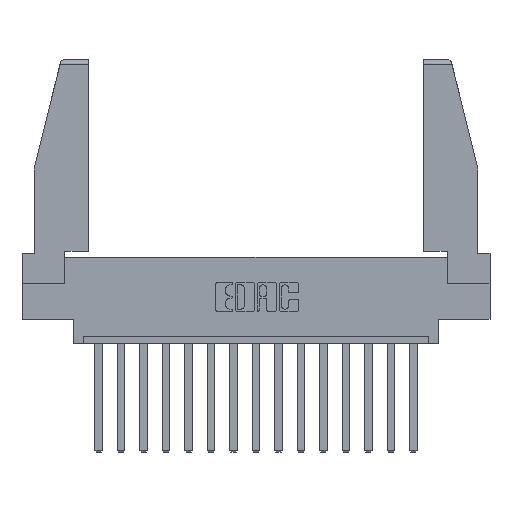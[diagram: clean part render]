
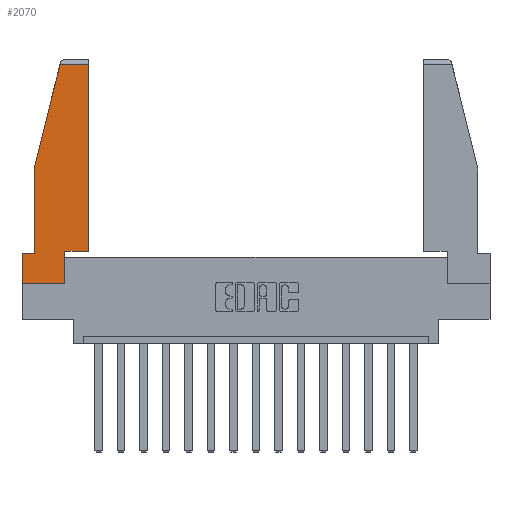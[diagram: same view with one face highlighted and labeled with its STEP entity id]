
A CAD part, top view. The second image highlights one B-rep face of the part: STEP entity #2070.
In plain terms, the highlighted planar face has unit normal (0, 0, 1).
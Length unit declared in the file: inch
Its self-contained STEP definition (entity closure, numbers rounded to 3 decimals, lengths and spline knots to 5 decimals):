
#109 = AXIS2_PLACEMENT_3D ( 'NONE', #7690, #15931, #11987 ) ;
#240 = EDGE_CURVE ( 'NONE', #331, #1604, #15141, .T. ) ;
#331 = VERTEX_POINT ( 'NONE', #11324 ) ;
#376 = LINE ( 'NONE', #4694, #9643 ) ;
#450 = DIRECTION ( 'NONE',  ( 1., 0., 0. ) ) ;
#595 = VERTEX_POINT ( 'NONE', #5426 ) ;
#1354 = VERTEX_POINT ( 'NONE', #14754 ) ;
#1604 = VERTEX_POINT ( 'NONE', #13686 ) ;
#1904 = VERTEX_POINT ( 'NONE', #2122 ) ;
#2070 = ADVANCED_FACE ( 'NONE', ( #9452 ), #15615, .T. ) ;
#2122 = CARTESIAN_POINT ( 'NONE',  ( 0.086, 0.8, 0. ) ) ;
#2457 = EDGE_CURVE ( 'NONE', #1354, #1904, #376, .T. ) ;
#2693 = VECTOR ( 'NONE', #16957, 39.37008 ) ;
#2701 = EDGE_CURVE ( 'NONE', #1604, #8536, #5945, .T. ) ;
#2805 = ORIENTED_EDGE ( 'NONE', *, *, #3983, .T. ) ;
#3737 = DIRECTION ( 'NONE',  ( 0., 1., 0. ) ) ;
#3796 = CARTESIAN_POINT ( 'NONE',  ( 0., 0.21, 0. ) ) ;
#3983 = EDGE_CURVE ( 'NONE', #12000, #1354, #9051, .T. ) ;
#4038 = ORIENTED_EDGE ( 'NONE', *, *, #7397, .T. ) ;
#4281 = ORIENTED_EDGE ( 'NONE', *, *, #14406, .T. ) ;
#4411 = ORIENTED_EDGE ( 'NONE', *, *, #2701, .T. ) ;
#4694 = CARTESIAN_POINT ( 'NONE',  ( 0.271, 1.55, 0. ) ) ;
#5068 = ORIENTED_EDGE ( 'NONE', *, *, #2457, .T. ) ;
#5155 = CARTESIAN_POINT ( 'NONE',  ( 0.297, 0.223, 0. ) ) ;
#5426 = CARTESIAN_POINT ( 'NONE',  ( 0., 0.21, 0. ) ) ;
#5733 = LINE ( 'NONE', #5155, #11703 ) ;
#5945 = LINE ( 'NONE', #13272, #7174 ) ;
#6306 = DIRECTION ( 'NONE',  ( -1., 0., 0. ) ) ;
#7025 = DIRECTION ( 'NONE',  ( -0.239, -0.971, 0. ) ) ;
#7174 = VECTOR ( 'NONE', #8044, 39.37008 ) ;
#7397 = EDGE_CURVE ( 'NONE', #9286, #595, #16589, .T. ) ;
#7690 = CARTESIAN_POINT ( 'NONE',  ( 0., 0., 0. ) ) ;
#8044 = DIRECTION ( 'NONE',  ( 0., 1., 0. ) ) ;
#8536 = VERTEX_POINT ( 'NONE', #11276 ) ;
#8558 = DIRECTION ( 'NONE',  ( 0., -1., 0. ) ) ;
#9051 = LINE ( 'NONE', #13039, #2693 ) ;
#9180 = CARTESIAN_POINT ( 'NONE',  ( 0., 0.21, 0. ) ) ;
#9286 = VERTEX_POINT ( 'NONE', #13851 ) ;
#9452 = FACE_OUTER_BOUND ( 'NONE', #16205, .T. ) ;
#9643 = VECTOR ( 'NONE', #7025, 39.37008 ) ;
#10117 = LINE ( 'NONE', #9180, #16724 ) ;
#10255 = CARTESIAN_POINT ( 'NONE',  ( 0.461, 1.52, 0. ) ) ;
#10684 = VERTEX_POINT ( 'NONE', #12707 ) ;
#10773 = ORIENTED_EDGE ( 'NONE', *, *, #240, .T. ) ;
#10779 = VECTOR ( 'NONE', #450, 39.37008 ) ;
#11276 = CARTESIAN_POINT ( 'NONE',  ( 0.297, 0.223, 0. ) ) ;
#11324 = CARTESIAN_POINT ( 'NONE',  ( 0., 0., 0. ) ) ;
#11566 = LINE ( 'NONE', #11645, #12801 ) ;
#11645 = CARTESIAN_POINT ( 'NONE',  ( 0.461, 0.223, 0. ) ) ;
#11703 = VECTOR ( 'NONE', #13034, 39.37008 ) ;
#11987 = DIRECTION ( 'NONE',  ( 1., 0., 0. ) ) ;
#12000 = VERTEX_POINT ( 'NONE', #10255 ) ;
#12104 = DIRECTION ( 'NONE',  ( 0., -1., 0. ) ) ;
#12196 = CARTESIAN_POINT ( 'NONE',  ( 0., 0., 0. ) ) ;
#12595 = LINE ( 'NONE', #13732, #13425 ) ;
#12707 = CARTESIAN_POINT ( 'NONE',  ( 0.461, 0.223, 0. ) ) ;
#12801 = VECTOR ( 'NONE', #3737, 39.37008 ) ;
#13034 = DIRECTION ( 'NONE',  ( 1., 0., 0. ) ) ;
#13039 = CARTESIAN_POINT ( 'NONE',  ( 0., 1.52, 0. ) ) ;
#13272 = CARTESIAN_POINT ( 'NONE',  ( 0.297, 0., 0. ) ) ;
#13425 = VECTOR ( 'NONE', #8558, 39.37008 ) ;
#13686 = CARTESIAN_POINT ( 'NONE',  ( 0.297, 0., 0. ) ) ;
#13732 = CARTESIAN_POINT ( 'NONE',  ( 0.086, 0.8, 0. ) ) ;
#13851 = CARTESIAN_POINT ( 'NONE',  ( 0.086, 0.21, 0. ) ) ;
#14406 = EDGE_CURVE ( 'NONE', #1904, #9286, #12595, .T. ) ;
#14600 = EDGE_CURVE ( 'NONE', #10684, #12000, #11566, .T. ) ;
#14662 = ORIENTED_EDGE ( 'NONE', *, *, #14600, .T. ) ;
#14754 = CARTESIAN_POINT ( 'NONE',  ( 0.2636, 1.52, 0. ) ) ;
#14838 = EDGE_CURVE ( 'NONE', #595, #331, #10117, .T. ) ;
#14958 = ORIENTED_EDGE ( 'NONE', *, *, #14838, .T. ) ;
#15141 = LINE ( 'NONE', #12196, #10779 ) ;
#15180 = ORIENTED_EDGE ( 'NONE', *, *, #16270, .T. ) ;
#15372 = VECTOR ( 'NONE', #6306, 39.37008 ) ;
#15615 = PLANE ( 'NONE',  #109 ) ;
#15931 = DIRECTION ( 'NONE',  ( 0., 0., 1. ) ) ;
#16205 = EDGE_LOOP ( 'NONE', ( #14662, #2805, #5068, #4281, #4038, #14958, #10773, #4411, #15180 ) ) ;
#16270 = EDGE_CURVE ( 'NONE', #8536, #10684, #5733, .T. ) ;
#16589 = LINE ( 'NONE', #3796, #15372 ) ;
#16724 = VECTOR ( 'NONE', #12104, 39.37008 ) ;
#16957 = DIRECTION ( 'NONE',  ( -1., 0., 0. ) ) ;
